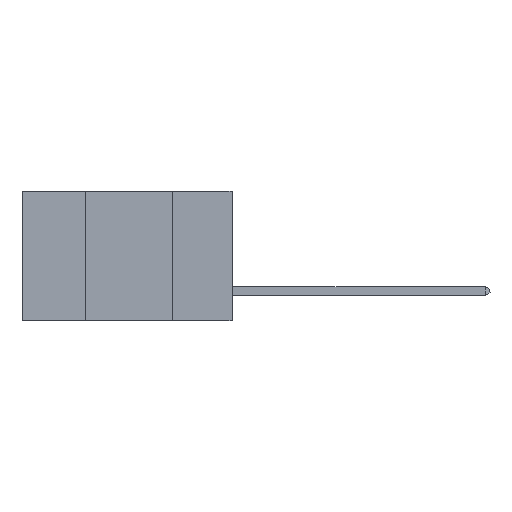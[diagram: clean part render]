
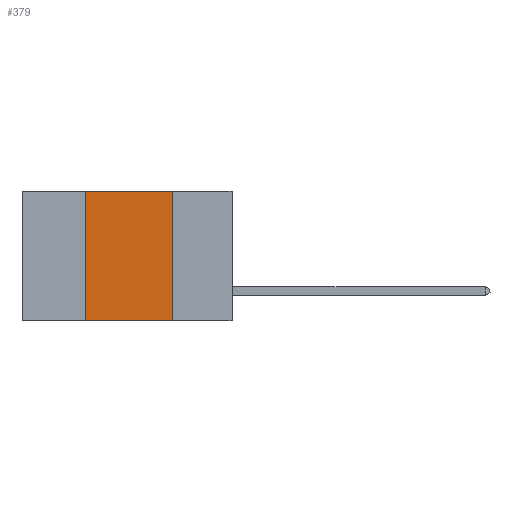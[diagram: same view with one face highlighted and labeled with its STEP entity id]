
A CAD part, left-side view. The second image highlights one B-rep face of the part: STEP entity #379.
In plain terms, the highlighted planar face has unit normal (-1, 0, 0).
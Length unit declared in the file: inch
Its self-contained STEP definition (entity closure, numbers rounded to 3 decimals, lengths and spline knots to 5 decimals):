
#379 = ADVANCED_FACE ( 'NONE', ( #12397 ), #5325, .F. ) ;
#648 = VERTEX_POINT ( 'NONE', #13308 ) ;
#1097 = CARTESIAN_POINT ( 'NONE',  ( 0., 0.6, 0. ) ) ;
#1154 = EDGE_CURVE ( 'NONE', #648, #11684, #8261, .T. ) ;
#1241 = DIRECTION ( 'NONE',  ( 1., 0., 0. ) ) ;
#1728 = DIRECTION ( 'NONE',  ( 0., 0., 1. ) ) ;
#1780 = VECTOR ( 'NONE', #10543, 39.37008 ) ;
#1794 = ORIENTED_EDGE ( 'NONE', *, *, #12389, .T. ) ;
#2046 = DIRECTION ( 'NONE',  ( 0., 0., -1. ) ) ;
#2295 = CARTESIAN_POINT ( 'NONE',  ( 0., 0.6, 0. ) ) ;
#2502 = VECTOR ( 'NONE', #1728, 39.37008 ) ;
#2573 = CARTESIAN_POINT ( 'NONE',  ( 0., 0.17, 0. ) ) ;
#2800 = VERTEX_POINT ( 'NONE', #7424 ) ;
#2961 = EDGE_CURVE ( 'NONE', #12368, #2800, #5733, .T. ) ;
#3752 = ORIENTED_EDGE ( 'NONE', *, *, #1154, .F. ) ;
#4552 = CARTESIAN_POINT ( 'NONE',  ( 0., 0.6, -0.37 ) ) ;
#5325 = PLANE ( 'NONE',  #7249 ) ;
#5733 = LINE ( 'NONE', #5797, #8684 ) ;
#5797 = CARTESIAN_POINT ( 'NONE',  ( 0., 0.17, 0. ) ) ;
#6392 = LINE ( 'NONE', #2295, #1780 ) ;
#6534 = ORIENTED_EDGE ( 'NONE', *, *, #2961, .F. ) ;
#7086 = EDGE_CURVE ( 'NONE', #11684, #12368, #6392, .T. ) ;
#7249 = AXIS2_PLACEMENT_3D ( 'NONE', #1097, #1241, #2046 ) ;
#7424 = CARTESIAN_POINT ( 'NONE',  ( 0., 0.17, -0.37 ) ) ;
#7537 = VECTOR ( 'NONE', #12973, 39.37008 ) ;
#8261 = LINE ( 'NONE', #10120, #2502 ) ;
#8684 = VECTOR ( 'NONE', #12998, 39.37008 ) ;
#8838 = LINE ( 'NONE', #4552, #7537 ) ;
#10120 = CARTESIAN_POINT ( 'NONE',  ( 0., 0.42, 0. ) ) ;
#10543 = DIRECTION ( 'NONE',  ( 0., -1., 0. ) ) ;
#11684 = VERTEX_POINT ( 'NONE', #12459 ) ;
#12193 = EDGE_LOOP ( 'NONE', ( #6534, #12557, #3752, #1794 ) ) ;
#12368 = VERTEX_POINT ( 'NONE', #2573 ) ;
#12389 = EDGE_CURVE ( 'NONE', #648, #2800, #8838, .T. ) ;
#12397 = FACE_OUTER_BOUND ( 'NONE', #12193, .T. ) ;
#12459 = CARTESIAN_POINT ( 'NONE',  ( 0., 0.42, 0. ) ) ;
#12557 = ORIENTED_EDGE ( 'NONE', *, *, #7086, .F. ) ;
#12973 = DIRECTION ( 'NONE',  ( 0., -1., 0. ) ) ;
#12998 = DIRECTION ( 'NONE',  ( 0., 0., -1. ) ) ;
#13308 = CARTESIAN_POINT ( 'NONE',  ( 0., 0.42, -0.37 ) ) ;
